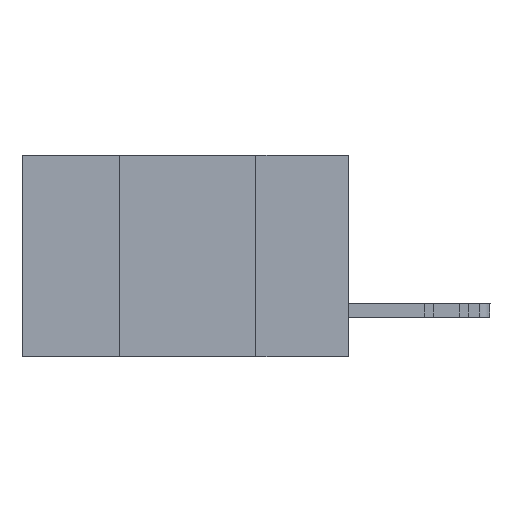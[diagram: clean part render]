
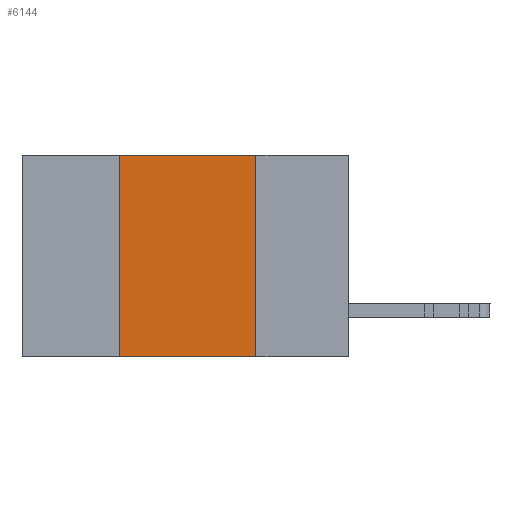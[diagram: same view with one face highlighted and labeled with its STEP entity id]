
A CAD part, left-side view. The second image highlights one B-rep face of the part: STEP entity #6144.
In plain terms, the highlighted planar face has unit normal (-1, 0, 0).
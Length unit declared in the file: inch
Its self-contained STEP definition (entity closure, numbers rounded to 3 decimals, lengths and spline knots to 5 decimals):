
#844 = VECTOR ( 'NONE', #17756, 39.37008 ) ;
#2843 = CARTESIAN_POINT ( 'NONE',  ( 0., 0.17, 0. ) ) ;
#2950 = ORIENTED_EDGE ( 'NONE', *, *, #5574, .T. ) ;
#3484 = VERTEX_POINT ( 'NONE', #17148 ) ;
#3707 = EDGE_LOOP ( 'NONE', ( #4802, #8702, #4286, #2950 ) ) ;
#4183 = VECTOR ( 'NONE', #10078, 39.37008 ) ;
#4286 = ORIENTED_EDGE ( 'NONE', *, *, #16074, .F. ) ;
#4802 = ORIENTED_EDGE ( 'NONE', *, *, #9060, .F. ) ;
#5574 = EDGE_CURVE ( 'NONE', #3484, #21978, #19009, .T. ) ;
#6144 = ADVANCED_FACE ( 'NONE', ( #11118 ), #22020, .F. ) ;
#8109 = CARTESIAN_POINT ( 'NONE',  ( 0., 0.42, -0.37 ) ) ;
#8418 = DIRECTION ( 'NONE',  ( 0., 0., 1. ) ) ;
#8702 = ORIENTED_EDGE ( 'NONE', *, *, #20650, .F. ) ;
#9060 = EDGE_CURVE ( 'NONE', #22135, #21978, #18080, .T. ) ;
#10078 = DIRECTION ( 'NONE',  ( 0., 0., -1. ) ) ;
#10849 = CARTESIAN_POINT ( 'NONE',  ( 0., 0.17, -0.37 ) ) ;
#11118 = FACE_OUTER_BOUND ( 'NONE', #3707, .T. ) ;
#11440 = VERTEX_POINT ( 'NONE', #16957 ) ;
#14434 = VECTOR ( 'NONE', #18047, 39.37008 ) ;
#16074 = EDGE_CURVE ( 'NONE', #3484, #11440, #18239, .T. ) ;
#16332 = CARTESIAN_POINT ( 'NONE',  ( 0., 0.17, -0.37 ) ) ;
#16957 = CARTESIAN_POINT ( 'NONE',  ( 0., 0.42, 0. ) ) ;
#17063 = CARTESIAN_POINT ( 'NONE',  ( 0., 0.6, -0.37 ) ) ;
#17148 = CARTESIAN_POINT ( 'NONE',  ( 0., 0.42, -0.37 ) ) ;
#17756 = DIRECTION ( 'NONE',  ( 0., -1., 0. ) ) ;
#18047 = DIRECTION ( 'NONE',  ( 0., -1., 0. ) ) ;
#18080 = LINE ( 'NONE', #10849, #4183 ) ;
#18239 = LINE ( 'NONE', #8109, #21658 ) ;
#18842 = LINE ( 'NONE', #21150, #844 ) ;
#19009 = LINE ( 'NONE', #17063, #14434 ) ;
#20238 = AXIS2_PLACEMENT_3D ( 'NONE', #21998, #22046, #22041 ) ;
#20650 = EDGE_CURVE ( 'NONE', #11440, #22135, #18842, .T. ) ;
#21150 = CARTESIAN_POINT ( 'NONE',  ( 0., 0.6, 0. ) ) ;
#21658 = VECTOR ( 'NONE', #8418, 39.37008 ) ;
#21978 = VERTEX_POINT ( 'NONE', #16332 ) ;
#21998 = CARTESIAN_POINT ( 'NONE',  ( 0., 0.6, 0. ) ) ;
#22020 = PLANE ( 'NONE',  #20238 ) ;
#22041 = DIRECTION ( 'NONE',  ( 0., 0., -1. ) ) ;
#22046 = DIRECTION ( 'NONE',  ( 1., 0., 0. ) ) ;
#22135 = VERTEX_POINT ( 'NONE', #2843 ) ;
